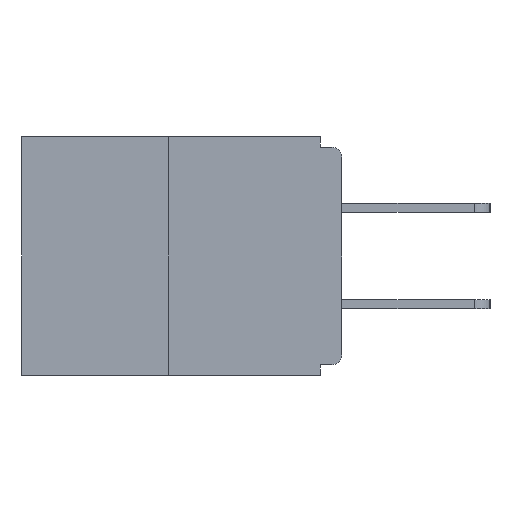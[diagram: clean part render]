
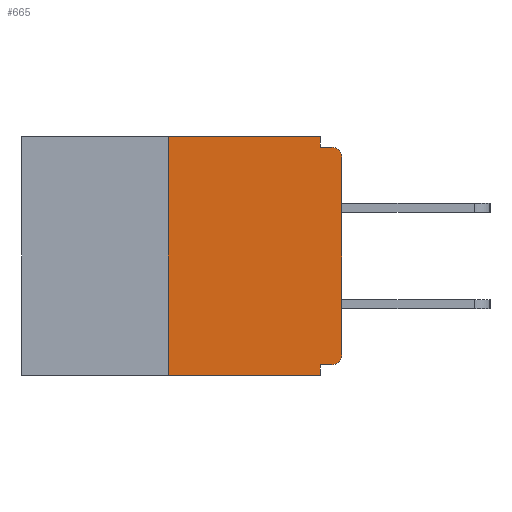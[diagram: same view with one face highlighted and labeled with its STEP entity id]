
A CAD part, left-side view. The second image highlights one B-rep face of the part: STEP entity #665.
In plain terms, the highlighted planar face has unit normal (-1, 0, 0).
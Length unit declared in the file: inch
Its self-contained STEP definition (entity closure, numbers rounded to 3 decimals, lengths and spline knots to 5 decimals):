
#223 = CARTESIAN_POINT ( 'NONE',  ( 0., 0., -0.015 ) ) ;
#665 = ADVANCED_FACE ( 'NONE', ( #14963 ), #7521, .F. ) ;
#799 = LINE ( 'NONE', #5814, #8939 ) ;
#899 = ORIENTED_EDGE ( 'NONE', *, *, #10385, .T. ) ;
#1636 = LINE ( 'NONE', #223, #10552 ) ;
#2112 = EDGE_CURVE ( 'NONE', #11467, #13660, #799, .T. ) ;
#2204 = ORIENTED_EDGE ( 'NONE', *, *, #2112, .T. ) ;
#2343 = VECTOR ( 'NONE', #12437, 39.37008 ) ;
#2602 = EDGE_CURVE ( 'NONE', #12645, #11467, #10601, .T. ) ;
#2719 = AXIS2_PLACEMENT_3D ( 'NONE', #6452, #5395, #13575 ) ;
#3127 = VERTEX_POINT ( 'NONE', #7868 ) ;
#3247 = LINE ( 'NONE', #12409, #4321 ) ;
#3294 = DIRECTION ( 'NONE',  ( -1., 0., 0. ) ) ;
#3801 = EDGE_LOOP ( 'NONE', ( #7895, #10163, #899, #7560, #13264, #4364, #2204, #5759, #8545, #5905 ) ) ;
#4193 = CARTESIAN_POINT ( 'NONE',  ( 0., 0.015, -0.328 ) ) ;
#4321 = VECTOR ( 'NONE', #9969, 39.37008 ) ;
#4364 = ORIENTED_EDGE ( 'NONE', *, *, #2602, .T. ) ;
#4831 = DIRECTION ( 'NONE',  ( 0., 1., 0. ) ) ;
#5020 = AXIS2_PLACEMENT_3D ( 'NONE', #10245, #3294, #6635 ) ;
#5395 = DIRECTION ( 'NONE',  ( 1., 0., 0. ) ) ;
#5401 = LINE ( 'NONE', #6288, #2343 ) ;
#5414 = LINE ( 'NONE', #9380, #13982 ) ;
#5479 = CARTESIAN_POINT ( 'NONE',  ( 0., 0.015, -0.313 ) ) ;
#5759 = ORIENTED_EDGE ( 'NONE', *, *, #8319, .T. ) ;
#5814 = CARTESIAN_POINT ( 'NONE',  ( 0., 0., 0. ) ) ;
#5905 = ORIENTED_EDGE ( 'NONE', *, *, #12907, .F. ) ;
#5958 = LINE ( 'NONE', #11383, #11825 ) ;
#6124 = VECTOR ( 'NONE', #11347, 39.37008 ) ;
#6288 = CARTESIAN_POINT ( 'NONE',  ( 0., 0.031, -0.343 ) ) ;
#6329 = VERTEX_POINT ( 'NONE', #9592 ) ;
#6452 = CARTESIAN_POINT ( 'NONE',  ( 0., 0.46, 0. ) ) ;
#6635 = DIRECTION ( 'NONE',  ( 0., 0., -1. ) ) ;
#7521 = PLANE ( 'NONE',  #2719 ) ;
#7560 = ORIENTED_EDGE ( 'NONE', *, *, #10967, .F. ) ;
#7576 = LINE ( 'NONE', #11317, #6124 ) ;
#7708 = CARTESIAN_POINT ( 'NONE',  ( 0., 0.031, 0. ) ) ;
#7868 = CARTESIAN_POINT ( 'NONE',  ( 0., 0.031, -0.328 ) ) ;
#7895 = ORIENTED_EDGE ( 'NONE', *, *, #13856, .F. ) ;
#8115 = CARTESIAN_POINT ( 'NONE',  ( 0., 0.25, -0.343 ) ) ;
#8205 = CIRCLE ( 'NONE', #5020, 0.015 ) ;
#8319 = EDGE_CURVE ( 'NONE', #13660, #9178, #8205, .T. ) ;
#8545 = ORIENTED_EDGE ( 'NONE', *, *, #10675, .F. ) ;
#8816 = EDGE_CURVE ( 'NONE', #12645, #3127, #11152, .T. ) ;
#8939 = VECTOR ( 'NONE', #9176, 39.37008 ) ;
#8951 = VERTEX_POINT ( 'NONE', #13248 ) ;
#9043 = DIRECTION ( 'NONE',  ( 0., 0., -1. ) ) ;
#9165 = CARTESIAN_POINT ( 'NONE',  ( 0., 0.031, -0.343 ) ) ;
#9176 = DIRECTION ( 'NONE',  ( 0., 0., 1. ) ) ;
#9178 = VERTEX_POINT ( 'NONE', #12908 ) ;
#9299 = VERTEX_POINT ( 'NONE', #8115 ) ;
#9380 = CARTESIAN_POINT ( 'NONE',  ( 0., 0.25, 0. ) ) ;
#9592 = CARTESIAN_POINT ( 'NONE',  ( 0., 0.25, 0. ) ) ;
#9911 = EDGE_CURVE ( 'NONE', #9299, #6329, #5414, .T. ) ;
#9969 = DIRECTION ( 'NONE',  ( 0., -1., 0. ) ) ;
#10163 = ORIENTED_EDGE ( 'NONE', *, *, #9911, .F. ) ;
#10245 = CARTESIAN_POINT ( 'NONE',  ( 0., 0.015, -0.03 ) ) ;
#10385 = EDGE_CURVE ( 'NONE', #9299, #10457, #7576, .T. ) ;
#10417 = DIRECTION ( 'NONE',  ( 0., 0., 1. ) ) ;
#10457 = VERTEX_POINT ( 'NONE', #9165 ) ;
#10552 = VECTOR ( 'NONE', #10623, 39.37008 ) ;
#10601 = CIRCLE ( 'NONE', #14688, 0.015 ) ;
#10623 = DIRECTION ( 'NONE',  ( 0., -1., 0. ) ) ;
#10675 = EDGE_CURVE ( 'NONE', #8951, #9178, #1636, .T. ) ;
#10917 = CARTESIAN_POINT ( 'NONE',  ( 0., 0., -0.313 ) ) ;
#10967 = EDGE_CURVE ( 'NONE', #3127, #10457, #5401, .T. ) ;
#11043 = VERTEX_POINT ( 'NONE', #7708 ) ;
#11152 = LINE ( 'NONE', #11839, #12408 ) ;
#11317 = CARTESIAN_POINT ( 'NONE',  ( 0., 0.46, -0.343 ) ) ;
#11347 = DIRECTION ( 'NONE',  ( 0., -1., 0. ) ) ;
#11383 = CARTESIAN_POINT ( 'NONE',  ( 0., 0.031, 0. ) ) ;
#11467 = VERTEX_POINT ( 'NONE', #10917 ) ;
#11825 = VECTOR ( 'NONE', #9043, 39.37008 ) ;
#11839 = CARTESIAN_POINT ( 'NONE',  ( 0., 0., -0.328 ) ) ;
#12408 = VECTOR ( 'NONE', #4831, 39.37008 ) ;
#12409 = CARTESIAN_POINT ( 'NONE',  ( 0., 0.46, 0. ) ) ;
#12437 = DIRECTION ( 'NONE',  ( 0., 0., -1. ) ) ;
#12645 = VERTEX_POINT ( 'NONE', #4193 ) ;
#12907 = EDGE_CURVE ( 'NONE', #11043, #8951, #5958, .T. ) ;
#12908 = CARTESIAN_POINT ( 'NONE',  ( 0., 0.015, -0.015 ) ) ;
#13248 = CARTESIAN_POINT ( 'NONE',  ( 0., 0.031, -0.015 ) ) ;
#13264 = ORIENTED_EDGE ( 'NONE', *, *, #8816, .F. ) ;
#13575 = DIRECTION ( 'NONE',  ( 0., 0., -1. ) ) ;
#13660 = VERTEX_POINT ( 'NONE', #14134 ) ;
#13856 = EDGE_CURVE ( 'NONE', #6329, #11043, #3247, .T. ) ;
#13982 = VECTOR ( 'NONE', #10417, 39.37008 ) ;
#14134 = CARTESIAN_POINT ( 'NONE',  ( 0., 0., -0.03 ) ) ;
#14601 = DIRECTION ( 'NONE',  ( -1., 0., 0. ) ) ;
#14688 = AXIS2_PLACEMENT_3D ( 'NONE', #5479, #14601, #14806 ) ;
#14806 = DIRECTION ( 'NONE',  ( 0., 0., -1. ) ) ;
#14963 = FACE_OUTER_BOUND ( 'NONE', #3801, .T. ) ;
